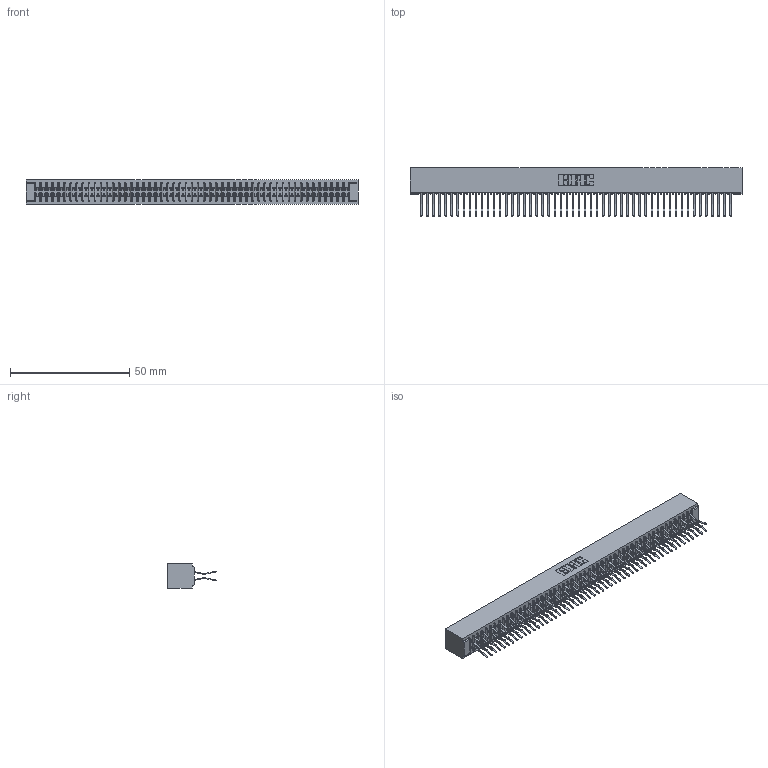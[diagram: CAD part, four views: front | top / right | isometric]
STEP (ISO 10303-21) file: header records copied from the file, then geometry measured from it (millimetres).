
FILE_DESCRIPTION (( 'STEP AP203' ), '1' );
FILE_NAME ('341-104-560-201.STEP', '2018-08-08T11:42:46', ( '' ), ( '' ), 'SwSTEP 2.0', 'SolidWorks 2016', '' );
FILE_SCHEMA (( 'CONFIG_CONTROL_DESIGN' ));
Length unit declared in the file: inch
Products named in the file (3): 341 Part_No Mounting Lugs; 341-292-001_341-292-160; 341-104-560-201
Assembly tree (105 placements, depth 2):
  341-104-560-201
    341 Part_No Mounting Lugs
    341-292-001_341-292-160  x104
Bounding box: 139.06 x 20.37 x 10.16 mm (x, y, z)
Volume: 10617.2 mm3; surface area: 20594.6 mm2
Topology: 105 solids, 105 shells, 7388 faces, 21456 edges, 13918 vertices
Faces by surface type: plane 4224, cylinder 2956, sphere 106, torus 102
Entity records: 61461 total; most frequent: CARTESIAN_POINT 10216, ORIENTED_EDGE 10152, DIRECTION 9910, EDGE_CURVE 5076, LINE 4110, VECTOR 4110, VERTEX_POINT 3206, AXIS2_PLACEMENT_3D 2900
